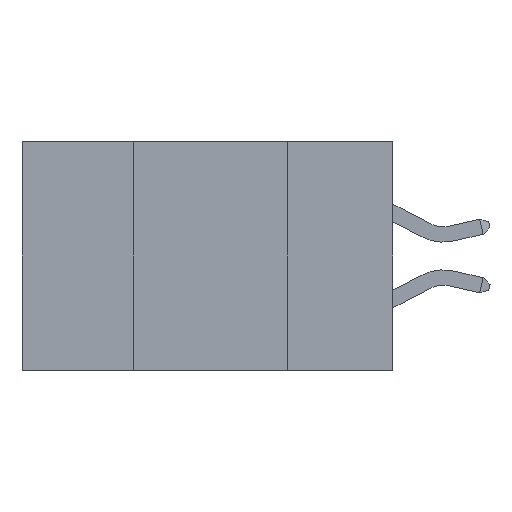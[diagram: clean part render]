
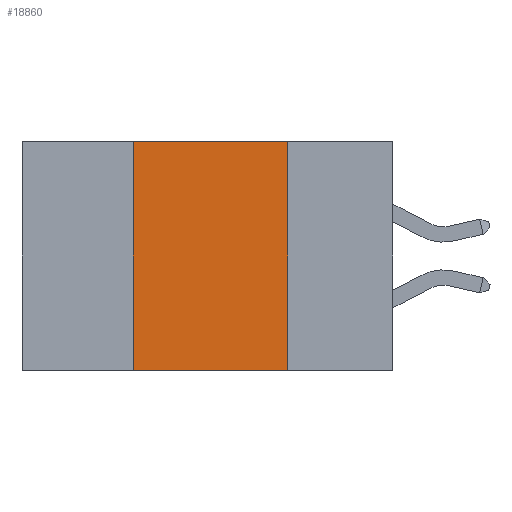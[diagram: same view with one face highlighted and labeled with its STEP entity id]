
A CAD part, left-side view. The second image highlights one B-rep face of the part: STEP entity #18860.
In plain terms, the highlighted planar face has unit normal (-1, 0, 0).
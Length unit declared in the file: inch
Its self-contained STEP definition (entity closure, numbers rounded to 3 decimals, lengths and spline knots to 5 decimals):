
#1724 = EDGE_CURVE ( 'NONE', #6840, #3400, #3715, .T. ) ;
#2931 = EDGE_LOOP ( 'NONE', ( #28141, #22992, #8275, #8027 ) ) ;
#3400 = VERTEX_POINT ( 'NONE', #4079 ) ;
#3715 = LINE ( 'NONE', #4409, #26673 ) ;
#4079 = CARTESIAN_POINT ( 'NONE',  ( 0., 0.17, 0. ) ) ;
#4409 = CARTESIAN_POINT ( 'NONE',  ( 0., 0.6, 0. ) ) ;
#4927 = CARTESIAN_POINT ( 'NONE',  ( 0., 0.17, -0.37 ) ) ;
#5504 = VECTOR ( 'NONE', #14422, 39.37008 ) ;
#6043 = EDGE_CURVE ( 'NONE', #3400, #25861, #14689, .T. ) ;
#6668 = DIRECTION ( 'NONE',  ( 0., 0., -1. ) ) ;
#6840 = VERTEX_POINT ( 'NONE', #9049 ) ;
#8027 = ORIENTED_EDGE ( 'NONE', *, *, #24873, .T. ) ;
#8275 = ORIENTED_EDGE ( 'NONE', *, *, #28292, .F. ) ;
#9049 = CARTESIAN_POINT ( 'NONE',  ( 0., 0.42, 0. ) ) ;
#9852 = VECTOR ( 'NONE', #6668, 39.37008 ) ;
#12431 = DIRECTION ( 'NONE',  ( 0., 0., -1. ) ) ;
#12716 = PLANE ( 'NONE',  #24207 ) ;
#12825 = LINE ( 'NONE', #21297, #5504 ) ;
#14422 = DIRECTION ( 'NONE',  ( 0., -1., 0. ) ) ;
#14562 = CARTESIAN_POINT ( 'NONE',  ( 0., 0.6, 0. ) ) ;
#14689 = LINE ( 'NONE', #15512, #9852 ) ;
#15512 = CARTESIAN_POINT ( 'NONE',  ( 0., 0.17, 0. ) ) ;
#15919 = CARTESIAN_POINT ( 'NONE',  ( 0., 0.42, -0.37 ) ) ;
#16994 = VERTEX_POINT ( 'NONE', #15919 ) ;
#17275 = CARTESIAN_POINT ( 'NONE',  ( 0., 0.42, 0. ) ) ;
#18860 = ADVANCED_FACE ( 'NONE', ( #28126 ), #12716, .F. ) ;
#19962 = DIRECTION ( 'NONE',  ( 0., -1., 0. ) ) ;
#20848 = LINE ( 'NONE', #17275, #27432 ) ;
#21297 = CARTESIAN_POINT ( 'NONE',  ( 0., 0.6, -0.37 ) ) ;
#22992 = ORIENTED_EDGE ( 'NONE', *, *, #1724, .F. ) ;
#24207 = AXIS2_PLACEMENT_3D ( 'NONE', #14562, #25715, #12431 ) ;
#24840 = DIRECTION ( 'NONE',  ( 0., 0., 1. ) ) ;
#24873 = EDGE_CURVE ( 'NONE', #16994, #25861, #12825, .T. ) ;
#25715 = DIRECTION ( 'NONE',  ( 1., 0., 0. ) ) ;
#25861 = VERTEX_POINT ( 'NONE', #4927 ) ;
#26673 = VECTOR ( 'NONE', #19962, 39.37008 ) ;
#27432 = VECTOR ( 'NONE', #24840, 39.37008 ) ;
#28126 = FACE_OUTER_BOUND ( 'NONE', #2931, .T. ) ;
#28141 = ORIENTED_EDGE ( 'NONE', *, *, #6043, .F. ) ;
#28292 = EDGE_CURVE ( 'NONE', #16994, #6840, #20848, .T. ) ;
